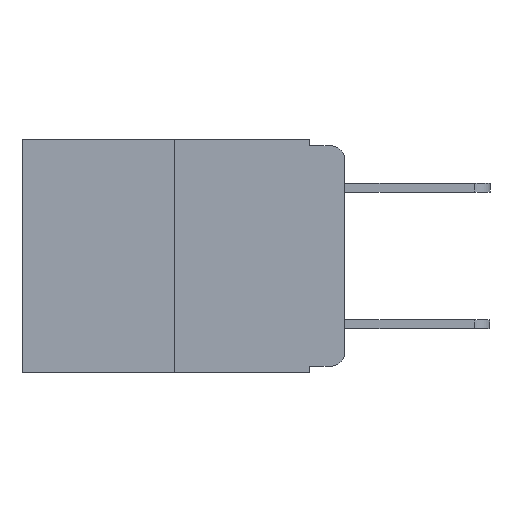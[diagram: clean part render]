
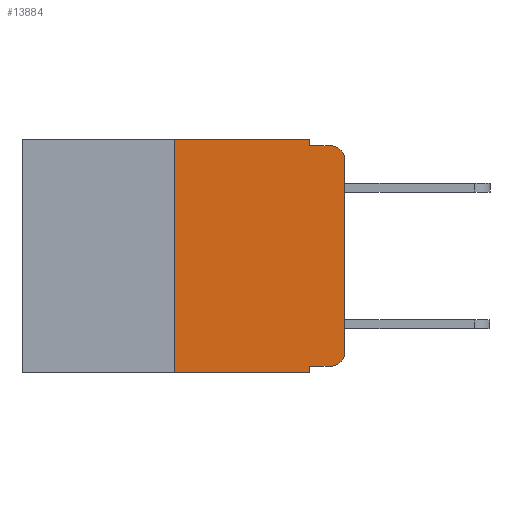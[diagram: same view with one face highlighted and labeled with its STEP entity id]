
A CAD part, left-side view. The second image highlights one B-rep face of the part: STEP entity #13884.
In plain terms, the highlighted planar face has unit normal (-1, 0, 0).
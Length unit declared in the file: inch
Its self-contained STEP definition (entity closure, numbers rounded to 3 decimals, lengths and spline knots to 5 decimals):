
#837 = VERTEX_POINT ( 'NONE', #6548 ) ;
#1232 = LINE ( 'NONE', #9055, #10155 ) ;
#1580 = DIRECTION ( 'NONE',  ( 0., 0., -1. ) ) ;
#1727 = VERTEX_POINT ( 'NONE', #17157 ) ;
#2073 = VECTOR ( 'NONE', #19657, 39.37008 ) ;
#2509 = AXIS2_PLACEMENT_3D ( 'NONE', #3663, #16035, #5448 ) ;
#3288 = PLANE ( 'NONE',  #14618 ) ;
#3327 = VERTEX_POINT ( 'NONE', #18290 ) ;
#3663 = CARTESIAN_POINT ( 'NONE',  ( 0., 0.02, -0.313 ) ) ;
#3689 = DIRECTION ( 'NONE',  ( 0., -1., 0. ) ) ;
#3865 = DIRECTION ( 'NONE',  ( 0., -1., 0. ) ) ;
#4066 = ORIENTED_EDGE ( 'NONE', *, *, #16897, .F. ) ;
#4303 = VECTOR ( 'NONE', #21479, 39.37008 ) ;
#4681 = LINE ( 'NONE', #16274, #22744 ) ;
#4761 = VERTEX_POINT ( 'NONE', #9635 ) ;
#4810 = CARTESIAN_POINT ( 'NONE',  ( 0., 0.25, -0.343 ) ) ;
#4947 = VERTEX_POINT ( 'NONE', #4810 ) ;
#4981 = VERTEX_POINT ( 'NONE', #22336 ) ;
#4985 = VECTOR ( 'NONE', #3865, 39.37008 ) ;
#5448 = DIRECTION ( 'NONE',  ( 0., 0., -1. ) ) ;
#5525 = CARTESIAN_POINT ( 'NONE',  ( 0., 0.051, 0. ) ) ;
#5749 = FACE_OUTER_BOUND ( 'NONE', #18703, .T. ) ;
#5773 = EDGE_CURVE ( 'NONE', #4947, #3327, #11523, .T. ) ;
#6010 = ORIENTED_EDGE ( 'NONE', *, *, #11441, .T. ) ;
#6540 = EDGE_CURVE ( 'NONE', #837, #18293, #19919, .T. ) ;
#6548 = CARTESIAN_POINT ( 'NONE',  ( 0., 0., -0.03 ) ) ;
#6556 = CARTESIAN_POINT ( 'NONE',  ( 0., 0.473, 0. ) ) ;
#6623 = AXIS2_PLACEMENT_3D ( 'NONE', #18451, #7911, #20149 ) ;
#6796 = ORIENTED_EDGE ( 'NONE', *, *, #10134, .T. ) ;
#6863 = CARTESIAN_POINT ( 'NONE',  ( 0., 0.473, 0. ) ) ;
#7879 = VECTOR ( 'NONE', #14291, 39.37008 ) ;
#7911 = DIRECTION ( 'NONE',  ( -1., 0., 0. ) ) ;
#8021 = LINE ( 'NONE', #17987, #4985 ) ;
#8409 = VECTOR ( 'NONE', #20767, 39.37008 ) ;
#9055 = CARTESIAN_POINT ( 'NONE',  ( 0., 0.473, -0.343 ) ) ;
#9635 = CARTESIAN_POINT ( 'NONE',  ( 0., 0.051, -0.333 ) ) ;
#10134 = EDGE_CURVE ( 'NONE', #10271, #837, #13118, .T. ) ;
#10155 = VECTOR ( 'NONE', #3689, 39.37008 ) ;
#10271 = VERTEX_POINT ( 'NONE', #17994 ) ;
#10717 = ORIENTED_EDGE ( 'NONE', *, *, #16459, .F. ) ;
#11150 = LINE ( 'NONE', #6556, #20400 ) ;
#11215 = CARTESIAN_POINT ( 'NONE',  ( 0., 0.02, -0.01 ) ) ;
#11441 = EDGE_CURVE ( 'NONE', #1727, #10271, #18250, .T. ) ;
#11523 = LINE ( 'NONE', #21396, #2073 ) ;
#11913 = DIRECTION ( 'NONE',  ( 0., -1., 0. ) ) ;
#12108 = ORIENTED_EDGE ( 'NONE', *, *, #5773, .F. ) ;
#12183 = EDGE_CURVE ( 'NONE', #4761, #1727, #8021, .T. ) ;
#12204 = DIRECTION ( 'NONE',  ( 1., 0., 0. ) ) ;
#12837 = CARTESIAN_POINT ( 'NONE',  ( 0., 0.051, 0. ) ) ;
#13118 = LINE ( 'NONE', #22492, #8409 ) ;
#13471 = ORIENTED_EDGE ( 'NONE', *, *, #21463, .F. ) ;
#13884 = ADVANCED_FACE ( 'NONE', ( #5749 ), #3288, .F. ) ;
#14291 = DIRECTION ( 'NONE',  ( 0., 0., -1. ) ) ;
#14618 = AXIS2_PLACEMENT_3D ( 'NONE', #6863, #12204, #1580 ) ;
#15056 = CARTESIAN_POINT ( 'NONE',  ( 0., 0.051, -0.01 ) ) ;
#16035 = DIRECTION ( 'NONE',  ( -1., 0., 0. ) ) ;
#16274 = CARTESIAN_POINT ( 'NONE',  ( 0., 0.051, -0.01 ) ) ;
#16379 = EDGE_CURVE ( 'NONE', #4947, #19593, #1232, .T. ) ;
#16459 = EDGE_CURVE ( 'NONE', #4981, #20084, #18372, .T. ) ;
#16769 = ORIENTED_EDGE ( 'NONE', *, *, #19898, .F. ) ;
#16897 = EDGE_CURVE ( 'NONE', #4761, #19593, #17291, .T. ) ;
#17157 = CARTESIAN_POINT ( 'NONE',  ( 0., 0.02, -0.333 ) ) ;
#17291 = LINE ( 'NONE', #5525, #7879 ) ;
#17987 = CARTESIAN_POINT ( 'NONE',  ( 0., 0.051, -0.333 ) ) ;
#17994 = CARTESIAN_POINT ( 'NONE',  ( 0., 0., -0.313 ) ) ;
#18032 = DIRECTION ( 'NONE',  ( 0., -1., 0. ) ) ;
#18250 = CIRCLE ( 'NONE', #2509, 0.02 ) ;
#18290 = CARTESIAN_POINT ( 'NONE',  ( 0., 0.25, 0. ) ) ;
#18293 = VERTEX_POINT ( 'NONE', #11215 ) ;
#18372 = LINE ( 'NONE', #12837, #4303 ) ;
#18451 = CARTESIAN_POINT ( 'NONE',  ( 0., 0.02, -0.03 ) ) ;
#18703 = EDGE_LOOP ( 'NONE', ( #6796, #19956, #16769, #10717, #13471, #12108, #18938, #4066, #20822, #6010 ) ) ;
#18938 = ORIENTED_EDGE ( 'NONE', *, *, #16379, .T. ) ;
#19593 = VERTEX_POINT ( 'NONE', #20577 ) ;
#19657 = DIRECTION ( 'NONE',  ( 0., 0., 1. ) ) ;
#19898 = EDGE_CURVE ( 'NONE', #20084, #18293, #4681, .T. ) ;
#19919 = CIRCLE ( 'NONE', #6623, 0.02 ) ;
#19956 = ORIENTED_EDGE ( 'NONE', *, *, #6540, .T. ) ;
#20084 = VERTEX_POINT ( 'NONE', #15056 ) ;
#20149 = DIRECTION ( 'NONE',  ( 0., 0., -1. ) ) ;
#20400 = VECTOR ( 'NONE', #11913, 39.37008 ) ;
#20577 = CARTESIAN_POINT ( 'NONE',  ( 0., 0.051, -0.343 ) ) ;
#20767 = DIRECTION ( 'NONE',  ( 0., 0., 1. ) ) ;
#20822 = ORIENTED_EDGE ( 'NONE', *, *, #12183, .T. ) ;
#21396 = CARTESIAN_POINT ( 'NONE',  ( 0., 0.25, 0. ) ) ;
#21463 = EDGE_CURVE ( 'NONE', #3327, #4981, #11150, .T. ) ;
#21479 = DIRECTION ( 'NONE',  ( 0., 0., -1. ) ) ;
#22336 = CARTESIAN_POINT ( 'NONE',  ( 0., 0.051, 0. ) ) ;
#22492 = CARTESIAN_POINT ( 'NONE',  ( 0., 0., 0. ) ) ;
#22744 = VECTOR ( 'NONE', #18032, 39.37008 ) ;
